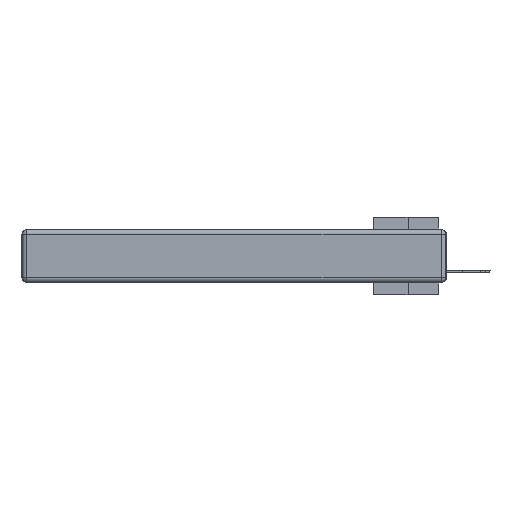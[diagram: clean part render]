
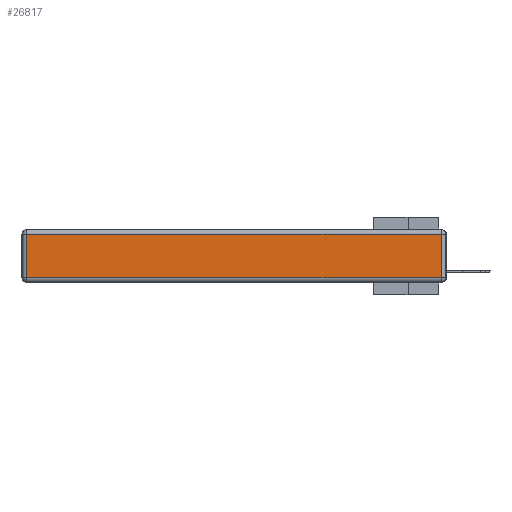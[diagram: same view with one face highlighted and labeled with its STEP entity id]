
A CAD part, left-side view. The second image highlights one B-rep face of the part: STEP entity #26817.
In plain terms, the highlighted planar face has unit normal (-1, 0, 0).
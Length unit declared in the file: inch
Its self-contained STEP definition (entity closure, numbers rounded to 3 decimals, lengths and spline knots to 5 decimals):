
#297 = CARTESIAN_POINT ( 'NONE',  ( 0., 0.03, -0.313 ) ) ;
#2242 = LINE ( 'NONE', #32934, #27468 ) ;
#2305 = DIRECTION ( 'NONE',  ( 0., 1., 0. ) ) ;
#3149 = EDGE_CURVE ( 'NONE', #12581, #3404, #19155, .T. ) ;
#3404 = VERTEX_POINT ( 'NONE', #35365 ) ;
#4960 = LINE ( 'NONE', #27681, #12158 ) ;
#5427 = CARTESIAN_POINT ( 'NONE',  ( 0., 0.03, -0.03 ) ) ;
#6587 = ORIENTED_EDGE ( 'NONE', *, *, #35340, .T. ) ;
#7148 = ORIENTED_EDGE ( 'NONE', *, *, #28387, .T. ) ;
#7598 = ORIENTED_EDGE ( 'NONE', *, *, #3149, .T. ) ;
#7734 = VERTEX_POINT ( 'NONE', #297 ) ;
#9847 = EDGE_LOOP ( 'NONE', ( #36347, #7148, #7598, #6587 ) ) ;
#12158 = VECTOR ( 'NONE', #33410, 39.37008 ) ;
#12578 = DIRECTION ( 'NONE',  ( 0., 0., 1. ) ) ;
#12581 = VERTEX_POINT ( 'NONE', #5427 ) ;
#13130 = FACE_OUTER_BOUND ( 'NONE', #9847, .T. ) ;
#15537 = CARTESIAN_POINT ( 'NONE',  ( 0., 0., -0.343 ) ) ;
#17256 = CARTESIAN_POINT ( 'NONE',  ( 0., 2.72, -0.313 ) ) ;
#19130 = CARTESIAN_POINT ( 'NONE',  ( 0., 0.03, -0.343 ) ) ;
#19155 = LINE ( 'NONE', #19691, #30807 ) ;
#19691 = CARTESIAN_POINT ( 'NONE',  ( 0., 2.75, -0.03 ) ) ;
#24220 = PLANE ( 'NONE',  #31018 ) ;
#24407 = DIRECTION ( 'NONE',  ( -1., 0., 0. ) ) ;
#25858 = VECTOR ( 'NONE', #32793, 39.37008 ) ;
#26371 = EDGE_CURVE ( 'NONE', #29422, #7734, #2242, .T. ) ;
#26817 = ADVANCED_FACE ( 'NONE', ( #13130 ), #24220, .T. ) ;
#27468 = VECTOR ( 'NONE', #29816, 39.37008 ) ;
#27681 = CARTESIAN_POINT ( 'NONE',  ( 0., 2.72, -0.343 ) ) ;
#28387 = EDGE_CURVE ( 'NONE', #7734, #12581, #32971, .T. ) ;
#29422 = VERTEX_POINT ( 'NONE', #17256 ) ;
#29816 = DIRECTION ( 'NONE',  ( 0., -1., 0. ) ) ;
#30807 = VECTOR ( 'NONE', #2305, 39.37008 ) ;
#31018 = AXIS2_PLACEMENT_3D ( 'NONE', #15537, #24407, #12578 ) ;
#32793 = DIRECTION ( 'NONE',  ( 0., 0., 1. ) ) ;
#32934 = CARTESIAN_POINT ( 'NONE',  ( 0., 0., -0.313 ) ) ;
#32971 = LINE ( 'NONE', #19130, #25858 ) ;
#33410 = DIRECTION ( 'NONE',  ( 0., 0., -1. ) ) ;
#35340 = EDGE_CURVE ( 'NONE', #3404, #29422, #4960, .T. ) ;
#35365 = CARTESIAN_POINT ( 'NONE',  ( 0., 2.72, -0.03 ) ) ;
#36347 = ORIENTED_EDGE ( 'NONE', *, *, #26371, .T. ) ;
